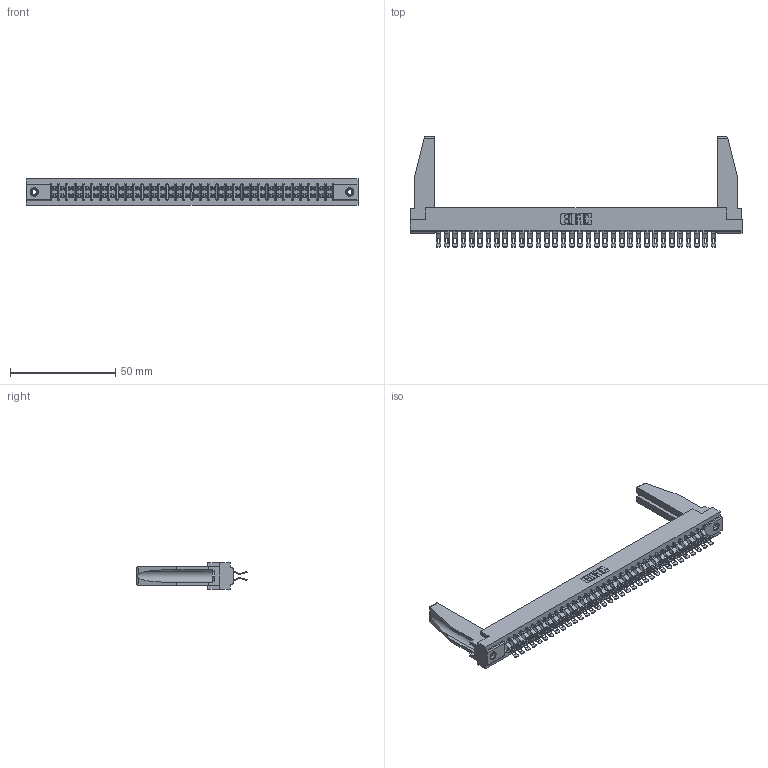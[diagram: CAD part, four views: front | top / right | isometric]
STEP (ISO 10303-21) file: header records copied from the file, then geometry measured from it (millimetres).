
FILE_DESCRIPTION (( 'STEP AP203' ), '1' );
FILE_NAME ('307-068-555-278.STEP', '2019-09-06T19:00:38', ( '' ), ( '' ), 'SwSTEP 2.0', 'SolidWorks 2016', '' );
FILE_SCHEMA (( 'CONFIG_CONTROL_DESIGN' ));
Length unit declared in the file: inch
Products named in the file (5): 307-068-555-278; 307 Part_.156 Dia Mounting Holes; 307-290-001_555; 307-220-078; 345-250-001_345-250-001-102
Assembly tree (73 placements, depth 2):
  307-068-555-278
    307 Part_.156 Dia Mounting Holes
    307-290-001_555  x68
    307-220-078  x2
    345-250-001_345-250-001-102  x2
Bounding box: 157.73 x 52.45 x 12.7 mm (x, y, z)
Volume: 20912.4 mm3; surface area: 25491 mm2
Topology: 73 solids, 73 shells, 4431 faces, 12961 edges, 8446 vertices
Faces by surface type: plane 2466, cylinder 1879, sphere 70, cone 12, torus 4
Entity records: 34198 total; most frequent: CARTESIAN_POINT 5612, ORIENTED_EDGE 5522, DIRECTION 5461, EDGE_CURVE 2761, LINE 2107, VECTOR 2107, VERTEX_POINT 1786, AXIS2_PLACEMENT_3D 1677
